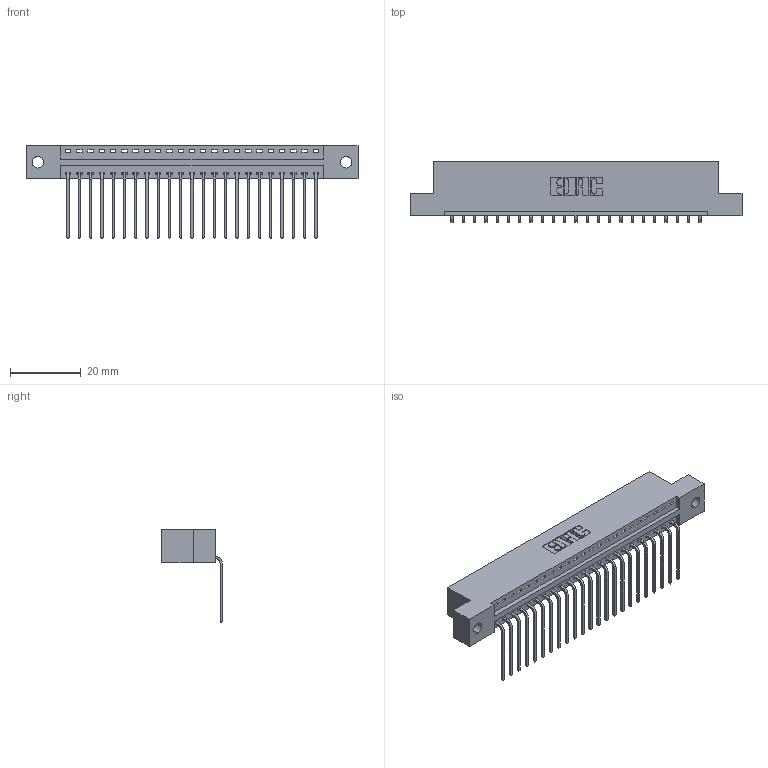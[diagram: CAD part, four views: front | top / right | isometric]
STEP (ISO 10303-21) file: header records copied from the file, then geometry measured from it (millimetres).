
FILE_DESCRIPTION (( 'STEP AP203' ), '1' );
FILE_NAME ('346-023-559-102.STEP', '2022-05-05T21:54:17', ( '' ), ( '' ), 'SwSTEP 2.0', 'SolidWorks 2020', '' );
FILE_SCHEMA (( 'CONFIG_CONTROL_DESIGN' ));
Length unit declared in the file: inch
Products named in the file (3): 346-023-559-102; 345-292-001_558 559 Tail - 1; 346 Part_Flush Mounting Lugs - 0.128 Dia
Assembly tree (24 placements, depth 2):
  346-023-559-102
    346 Part_Flush Mounting Lugs - 0.128 Dia
    345-292-001_558 559 Tail - 1  x23
Bounding box: 93.6 x 17.08 x 26.16 mm (x, y, z)
Volume: 8868.5 mm3; surface area: 11065.4 mm2
Topology: 24 solids, 24 shells, 1502 faces, 4515 edges, 2978 vertices
Faces by surface type: plane 1042, cylinder 460
Entity records: 16919 total; most frequent: CARTESIAN_POINT 2913, ORIENTED_EDGE 2870, DIRECTION 2593, EDGE_CURVE 1435, LINE 1211, VECTOR 1211, VERTEX_POINT 954, AXIS2_PLACEMENT_3D 691
